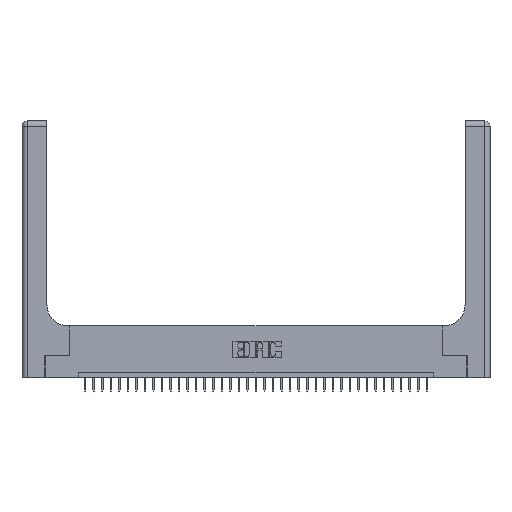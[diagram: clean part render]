
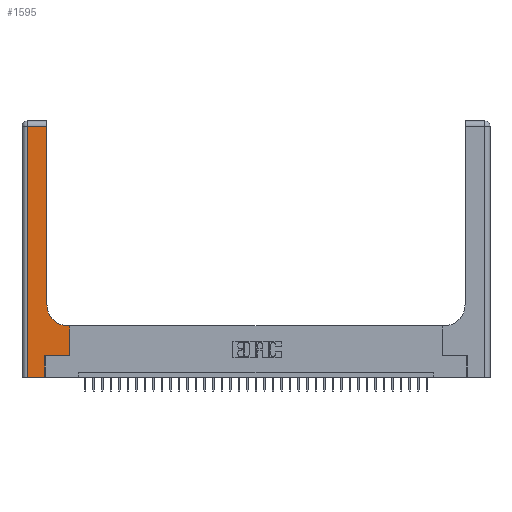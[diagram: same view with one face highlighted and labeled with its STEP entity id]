
A CAD part, top view. The second image highlights one B-rep face of the part: STEP entity #1595.
In plain terms, the highlighted planar face has unit normal (0, 0, 1).
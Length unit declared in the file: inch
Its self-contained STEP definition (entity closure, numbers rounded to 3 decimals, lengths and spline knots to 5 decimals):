
#41 = CARTESIAN_POINT ( 'NONE',  ( 0.2915, 3., 0.37 ) ) ;
#210 = LINE ( 'NONE', #6658, #23906 ) ;
#723 = CARTESIAN_POINT ( 'NONE',  ( 0.5415, 0.85, 0.37 ) ) ;
#852 = VERTEX_POINT ( 'NONE', #1715 ) ;
#1595 = ADVANCED_FACE ( 'NONE', ( #9217 ), #29825, .F. ) ;
#1715 = CARTESIAN_POINT ( 'NONE',  ( 0.2915, 0.85, 0.37 ) ) ;
#1760 = VERTEX_POINT ( 'NONE', #18707 ) ;
#2575 = DIRECTION ( 'NONE',  ( 0., 1., 0. ) ) ;
#2742 = VERTEX_POINT ( 'NONE', #8494 ) ;
#4346 = VECTOR ( 'NONE', #10813, 39.37008 ) ;
#5054 = DIRECTION ( 'NONE',  ( 0., 0., -1. ) ) ;
#6369 = EDGE_CURVE ( 'NONE', #24075, #2742, #25510, .T. ) ;
#6545 = VECTOR ( 'NONE', #17644, 39.37008 ) ;
#6658 = CARTESIAN_POINT ( 'NONE',  ( 0.06, 3., 0.37 ) ) ;
#7600 = ORIENTED_EDGE ( 'NONE', *, *, #30922, .T. ) ;
#7848 = LINE ( 'NONE', #7947, #4346 ) ;
#7947 = CARTESIAN_POINT ( 'NONE',  ( 0., 2.94, 0.37 ) ) ;
#7975 = VECTOR ( 'NONE', #27008, 39.37008 ) ;
#8016 = VERTEX_POINT ( 'NONE', #34921 ) ;
#8494 = CARTESIAN_POINT ( 'NONE',  ( 0.5585, 0.25, 0.37 ) ) ;
#9147 = CARTESIAN_POINT ( 'NONE',  ( 0.2915, 0.6, 0.37 ) ) ;
#9217 = FACE_OUTER_BOUND ( 'NONE', #19940, .T. ) ;
#9990 = CARTESIAN_POINT ( 'NONE',  ( 0.269, 0.25, 0.37 ) ) ;
#10696 = CARTESIAN_POINT ( 'NONE',  ( 0., 0., 0.37 ) ) ;
#10699 = AXIS2_PLACEMENT_3D ( 'NONE', #32860, #5054, #21802 ) ;
#10813 = DIRECTION ( 'NONE',  ( -1., 0., 0. ) ) ;
#11341 = VERTEX_POINT ( 'NONE', #32106 ) ;
#11420 = VERTEX_POINT ( 'NONE', #29036 ) ;
#11522 = EDGE_CURVE ( 'NONE', #852, #8016, #35156, .T. ) ;
#11971 = LINE ( 'NONE', #10696, #23838 ) ;
#12087 = ORIENTED_EDGE ( 'NONE', *, *, #27015, .T. ) ;
#12299 = LINE ( 'NONE', #9147, #6545 ) ;
#13439 = CARTESIAN_POINT ( 'NONE',  ( 0.269, 0., 0.37 ) ) ;
#14230 = CARTESIAN_POINT ( 'NONE',  ( 0.5585, 0.6, 0.37 ) ) ;
#14347 = DIRECTION ( 'NONE',  ( 0., 0., -1. ) ) ;
#14714 = CARTESIAN_POINT ( 'NONE',  ( 0.269, 0.25, 0.37 ) ) ;
#16100 = ORIENTED_EDGE ( 'NONE', *, *, #27827, .T. ) ;
#17644 = DIRECTION ( 'NONE',  ( -1., 0., 0. ) ) ;
#18707 = CARTESIAN_POINT ( 'NONE',  ( 0.06, 2.94, 0.37 ) ) ;
#18882 = LINE ( 'NONE', #23129, #28420 ) ;
#18984 = CIRCLE ( 'NONE', #26372, 0.25 ) ;
#19420 = CARTESIAN_POINT ( 'NONE',  ( 0.5585, 0.25, 0.37 ) ) ;
#19940 = EDGE_LOOP ( 'NONE', ( #21559, #26557, #16100, #26660, #7600, #31568, #21363, #34614, #12087 ) ) ;
#20380 = VECTOR ( 'NONE', #2575, 39.37008 ) ;
#21363 = ORIENTED_EDGE ( 'NONE', *, *, #25592, .T. ) ;
#21559 = ORIENTED_EDGE ( 'NONE', *, *, #11522, .T. ) ;
#21802 = DIRECTION ( 'NONE',  ( -1., 0., 0. ) ) ;
#22176 = EDGE_CURVE ( 'NONE', #8016, #1760, #7848, .T. ) ;
#23015 = LINE ( 'NONE', #19420, #20380 ) ;
#23129 = CARTESIAN_POINT ( 'NONE',  ( 0.269, 0., 0.37 ) ) ;
#23149 = VERTEX_POINT ( 'NONE', #13439 ) ;
#23838 = VECTOR ( 'NONE', #35644, 39.37008 ) ;
#23906 = VECTOR ( 'NONE', #26654, 39.37008 ) ;
#24075 = VERTEX_POINT ( 'NONE', #14714 ) ;
#25510 = LINE ( 'NONE', #9990, #7975 ) ;
#25592 = EDGE_CURVE ( 'NONE', #2742, #26948, #23015, .T. ) ;
#26372 = AXIS2_PLACEMENT_3D ( 'NONE', #723, #14347, #34010 ) ;
#26557 = ORIENTED_EDGE ( 'NONE', *, *, #22176, .T. ) ;
#26654 = DIRECTION ( 'NONE',  ( 0., -1., 0. ) ) ;
#26660 = ORIENTED_EDGE ( 'NONE', *, *, #28616, .T. ) ;
#26948 = VERTEX_POINT ( 'NONE', #14230 ) ;
#27008 = DIRECTION ( 'NONE',  ( 1., 0., 0. ) ) ;
#27015 = EDGE_CURVE ( 'NONE', #11420, #852, #18984, .T. ) ;
#27729 = VECTOR ( 'NONE', #28538, 39.37008 ) ;
#27827 = EDGE_CURVE ( 'NONE', #1760, #11341, #210, .T. ) ;
#28420 = VECTOR ( 'NONE', #31650, 39.37008 ) ;
#28538 = DIRECTION ( 'NONE',  ( 0., 1., 0. ) ) ;
#28616 = EDGE_CURVE ( 'NONE', #11341, #23149, #11971, .T. ) ;
#29036 = CARTESIAN_POINT ( 'NONE',  ( 0.5415, 0.6, 0.37 ) ) ;
#29825 = PLANE ( 'NONE',  #10699 ) ;
#30376 = EDGE_CURVE ( 'NONE', #26948, #11420, #12299, .T. ) ;
#30922 = EDGE_CURVE ( 'NONE', #23149, #24075, #18882, .T. ) ;
#31568 = ORIENTED_EDGE ( 'NONE', *, *, #6369, .T. ) ;
#31650 = DIRECTION ( 'NONE',  ( 0., 1., 0. ) ) ;
#32106 = CARTESIAN_POINT ( 'NONE',  ( 0.06, 0., 0.37 ) ) ;
#32860 = CARTESIAN_POINT ( 'NONE',  ( 0., 3., 0.37 ) ) ;
#34010 = DIRECTION ( 'NONE',  ( 1., 0., 0. ) ) ;
#34614 = ORIENTED_EDGE ( 'NONE', *, *, #30376, .T. ) ;
#34921 = CARTESIAN_POINT ( 'NONE',  ( 0.2915, 2.94, 0.37 ) ) ;
#35156 = LINE ( 'NONE', #41, #27729 ) ;
#35644 = DIRECTION ( 'NONE',  ( 1., 0., 0. ) ) ;
